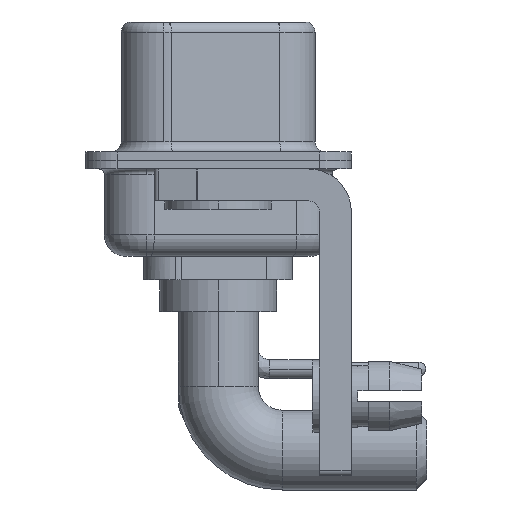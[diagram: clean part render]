
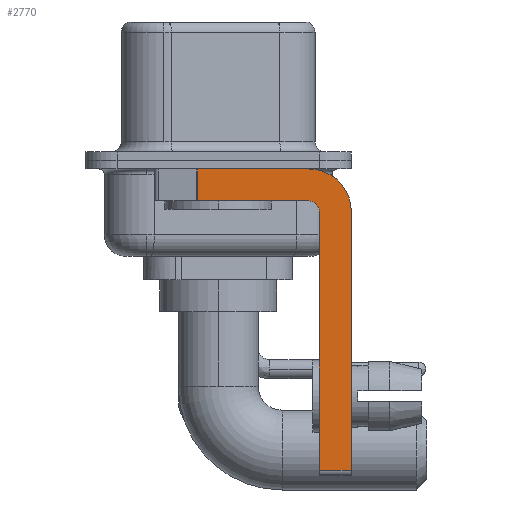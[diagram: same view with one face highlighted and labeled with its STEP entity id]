
A CAD part, left-side view. The second image highlights one B-rep face of the part: STEP entity #2770.
In plain terms, the highlighted planar face has unit normal (-1, 0, 0).
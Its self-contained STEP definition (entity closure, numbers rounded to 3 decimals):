
#386 = VERTEX_POINT ( 'NONE', #11981 ) ;
#1071 = VECTOR ( 'NONE', #13253, 1000. ) ;
#1192 = EDGE_CURVE ( 'NONE', #10839, #10564, #7843, .T. ) ;
#1214 = AXIS2_PLACEMENT_3D ( 'NONE', #3155, #5208, #13488 ) ;
#1323 = VECTOR ( 'NONE', #9552, 1000. ) ;
#2246 = CARTESIAN_POINT ( 'NONE',  ( -2.9, -4.25, -2.4 ) ) ;
#2755 = DIRECTION ( 'NONE',  ( 0., 0., 1. ) ) ;
#2770 = ADVANCED_FACE ( 'NONE', ( #10294 ), #25064, .F. ) ;
#3155 = CARTESIAN_POINT ( 'NONE',  ( -2.9, -4.25, -2.4 ) ) ;
#3316 = EDGE_CURVE ( 'NONE', #386, #6005, #12092, .T. ) ;
#3717 = VERTEX_POINT ( 'NONE', #26330 ) ;
#4606 = ORIENTED_EDGE ( 'NONE', *, *, #16556, .T. ) ;
#4618 = VECTOR ( 'NONE', #18277, 1000. ) ;
#4813 = CIRCLE ( 'NONE', #16505, 0.5 ) ;
#4921 = CARTESIAN_POINT ( 'NONE',  ( -2.9, -4.75, -14.55 ) ) ;
#5208 = DIRECTION ( 'NONE',  ( 1., 0., 0. ) ) ;
#5523 = CARTESIAN_POINT ( 'NONE',  ( -2.9, -4.25, -2.4 ) ) ;
#6005 = VERTEX_POINT ( 'NONE', #15281 ) ;
#6109 = VERTEX_POINT ( 'NONE', #7794 ) ;
#6325 = LINE ( 'NONE', #14604, #13930 ) ;
#6739 = LINE ( 'NONE', #25192, #1071 ) ;
#6813 = ORIENTED_EDGE ( 'NONE', *, *, #23946, .F. ) ;
#6814 = AXIS2_PLACEMENT_3D ( 'NONE', #2246, #8254, #24937 ) ;
#6852 = EDGE_CURVE ( 'NONE', #6109, #10839, #4813, .T. ) ;
#7598 = VECTOR ( 'NONE', #21213, 1000. ) ;
#7794 = CARTESIAN_POINT ( 'NONE',  ( -2.9, -4.75, -2.4 ) ) ;
#7843 = LINE ( 'NONE', #15979, #4618 ) ;
#8254 = DIRECTION ( 'NONE',  ( 1., 0., 0. ) ) ;
#8343 = CARTESIAN_POINT ( 'NONE',  ( -2.9, -6.25, -2.4 ) ) ;
#8603 = VERTEX_POINT ( 'NONE', #4921 ) ;
#9541 = ORIENTED_EDGE ( 'NONE', *, *, #25946, .T. ) ;
#9552 = DIRECTION ( 'NONE',  ( 0., -1., 0. ) ) ;
#9624 = CARTESIAN_POINT ( 'NONE',  ( -2.9, -4.25, -1.9 ) ) ;
#10294 = FACE_OUTER_BOUND ( 'NONE', #26221, .T. ) ;
#10564 = VERTEX_POINT ( 'NONE', #16536 ) ;
#10839 = VERTEX_POINT ( 'NONE', #9624 ) ;
#11519 = DIRECTION ( 'NONE',  ( -1., 0., 0. ) ) ;
#11648 = EDGE_CURVE ( 'NONE', #8603, #6109, #16880, .T. ) ;
#11925 = VERTEX_POINT ( 'NONE', #12744 ) ;
#11981 = CARTESIAN_POINT ( 'NONE',  ( -2.9, -4.25, -0.4 ) ) ;
#12092 = CIRCLE ( 'NONE', #1214, 2. ) ;
#12575 = EDGE_CURVE ( 'NONE', #6005, #11925, #14838, .T. ) ;
#12744 = CARTESIAN_POINT ( 'NONE',  ( -2.9, -6.25, -14.55 ) ) ;
#13253 = DIRECTION ( 'NONE',  ( 0., 0., -1. ) ) ;
#13349 = CARTESIAN_POINT ( 'NONE',  ( -2.9, -4.25, -14.55 ) ) ;
#13488 = DIRECTION ( 'NONE',  ( 0., 0., -1. ) ) ;
#13612 = LINE ( 'NONE', #13349, #1323 ) ;
#13930 = VECTOR ( 'NONE', #14735, 1000. ) ;
#14073 = VECTOR ( 'NONE', #2755, 1000. ) ;
#14604 = CARTESIAN_POINT ( 'NONE',  ( -2.9, 3., -0.4 ) ) ;
#14735 = DIRECTION ( 'NONE',  ( 0., -1., 0. ) ) ;
#14838 = LINE ( 'NONE', #8343, #7598 ) ;
#14849 = CARTESIAN_POINT ( 'NONE',  ( -2.9, -4.75, -14.8 ) ) ;
#15281 = CARTESIAN_POINT ( 'NONE',  ( -2.9, -6.25, -2.4 ) ) ;
#15979 = CARTESIAN_POINT ( 'NONE',  ( -2.9, -4.25, -1.9 ) ) ;
#16505 = AXIS2_PLACEMENT_3D ( 'NONE', #5523, #11519, #20047 ) ;
#16536 = CARTESIAN_POINT ( 'NONE',  ( -2.9, 0.978, -1.9 ) ) ;
#16556 = EDGE_CURVE ( 'NONE', #3717, #10564, #6739, .T. ) ;
#16880 = LINE ( 'NONE', #14849, #14073 ) ;
#18277 = DIRECTION ( 'NONE',  ( 0., 1., 0. ) ) ;
#18631 = ORIENTED_EDGE ( 'NONE', *, *, #3316, .F. ) ;
#18765 = ORIENTED_EDGE ( 'NONE', *, *, #12575, .F. ) ;
#20047 = DIRECTION ( 'NONE',  ( 0., 0., 1. ) ) ;
#20665 = ORIENTED_EDGE ( 'NONE', *, *, #1192, .F. ) ;
#21213 = DIRECTION ( 'NONE',  ( 0., 0., -1. ) ) ;
#23946 = EDGE_CURVE ( 'NONE', #3717, #386, #6325, .T. ) ;
#24665 = ORIENTED_EDGE ( 'NONE', *, *, #11648, .F. ) ;
#24937 = DIRECTION ( 'NONE',  ( 0., 0., -1. ) ) ;
#25064 = PLANE ( 'NONE',  #6814 ) ;
#25192 = CARTESIAN_POINT ( 'NONE',  ( -2.9, 0.978, -1.9 ) ) ;
#25687 = ORIENTED_EDGE ( 'NONE', *, *, #6852, .F. ) ;
#25946 = EDGE_CURVE ( 'NONE', #8603, #11925, #13612, .T. ) ;
#26221 = EDGE_LOOP ( 'NONE', ( #6813, #4606, #20665, #25687, #24665, #9541, #18765, #18631 ) ) ;
#26330 = CARTESIAN_POINT ( 'NONE',  ( -2.9, 0.978, -0.4 ) ) ;
